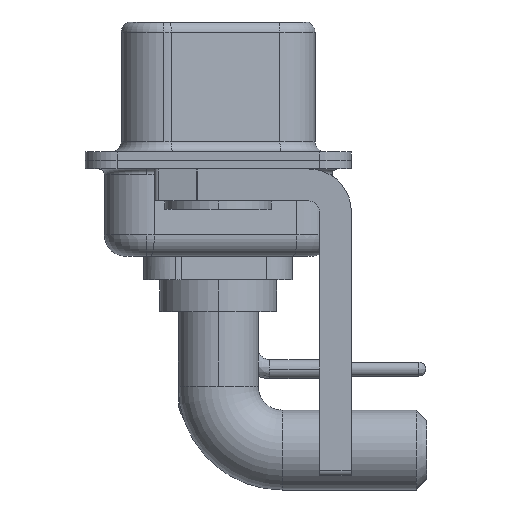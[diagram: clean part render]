
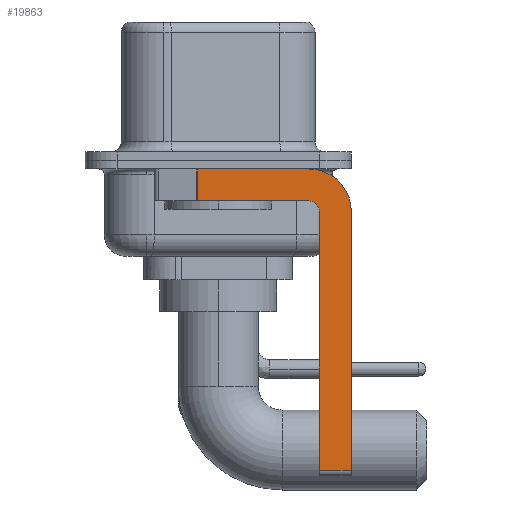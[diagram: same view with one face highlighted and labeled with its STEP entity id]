
A CAD part, left-side view. The second image highlights one B-rep face of the part: STEP entity #19863.
In plain terms, the highlighted planar face has unit normal (-1, 0, 0).
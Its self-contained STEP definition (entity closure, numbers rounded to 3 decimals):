
#294 = DIRECTION ( 'NONE',  ( 1., 0., 0. ) ) ;
#366 = CARTESIAN_POINT ( 'NONE',  ( -2.9, -6.25, -2.4 ) ) ;
#689 = DIRECTION ( 'NONE',  ( 0., 0., -1. ) ) ;
#1173 = VERTEX_POINT ( 'NONE', #2203 ) ;
#1324 = LINE ( 'NONE', #7914, #11558 ) ;
#1544 = VECTOR ( 'NONE', #7559, 1000. ) ;
#1708 = ORIENTED_EDGE ( 'NONE', *, *, #6287, .F. ) ;
#1928 = CARTESIAN_POINT ( 'NONE',  ( -2.9, -4.25, -2.4 ) ) ;
#2134 = CARTESIAN_POINT ( 'NONE',  ( -2.9, 0.978, -0.4 ) ) ;
#2203 = CARTESIAN_POINT ( 'NONE',  ( -2.9, -6.25, -14.55 ) ) ;
#2284 = LINE ( 'NONE', #5813, #1544 ) ;
#2319 = DIRECTION ( 'NONE',  ( 0., -1., 0. ) ) ;
#2606 = EDGE_CURVE ( 'NONE', #8714, #5023, #14496, .T. ) ;
#2607 = EDGE_CURVE ( 'NONE', #15973, #5023, #1324, .T. ) ;
#2671 = DIRECTION ( 'NONE',  ( 1., 0., 0. ) ) ;
#3146 = AXIS2_PLACEMENT_3D ( 'NONE', #1928, #15536, #5555 ) ;
#3405 = EDGE_CURVE ( 'NONE', #16512, #15973, #3497, .T. ) ;
#3497 = CIRCLE ( 'NONE', #3146, 0.5 ) ;
#3884 = CARTESIAN_POINT ( 'NONE',  ( -2.9, 3., -0.4 ) ) ;
#4293 = AXIS2_PLACEMENT_3D ( 'NONE', #10998, #2671, #689 ) ;
#4481 = LINE ( 'NONE', #6443, #9661 ) ;
#5023 = VERTEX_POINT ( 'NONE', #19657 ) ;
#5398 = EDGE_CURVE ( 'NONE', #10180, #1173, #12282, .T. ) ;
#5555 = DIRECTION ( 'NONE',  ( 0., 0., 1. ) ) ;
#5813 = CARTESIAN_POINT ( 'NONE',  ( -2.9, -6.25, -2.4 ) ) ;
#5873 = FACE_OUTER_BOUND ( 'NONE', #6847, .T. ) ;
#6287 = EDGE_CURVE ( 'NONE', #8714, #18024, #12193, .T. ) ;
#6347 = ORIENTED_EDGE ( 'NONE', *, *, #14965, .F. ) ;
#6420 = ORIENTED_EDGE ( 'NONE', *, *, #5398, .T. ) ;
#6443 = CARTESIAN_POINT ( 'NONE',  ( -2.9, -4.75, -14.8 ) ) ;
#6847 = EDGE_LOOP ( 'NONE', ( #1708, #19224, #11988, #19533, #14090, #6420, #12421, #6347 ) ) ;
#6906 = DIRECTION ( 'NONE',  ( 0., 0., -1. ) ) ;
#7509 = CARTESIAN_POINT ( 'NONE',  ( -2.9, -4.75, -14.55 ) ) ;
#7559 = DIRECTION ( 'NONE',  ( 0., 0., -1. ) ) ;
#7914 = CARTESIAN_POINT ( 'NONE',  ( -2.9, -4.25, -1.9 ) ) ;
#8714 = VERTEX_POINT ( 'NONE', #2134 ) ;
#9237 = CARTESIAN_POINT ( 'NONE',  ( -2.9, -4.25, -1.9 ) ) ;
#9661 = VECTOR ( 'NONE', #21037, 1000. ) ;
#9755 = DIRECTION ( 'NONE',  ( 0., 1., 0. ) ) ;
#10180 = VERTEX_POINT ( 'NONE', #7509 ) ;
#10998 = CARTESIAN_POINT ( 'NONE',  ( -2.9, -4.25, -2.4 ) ) ;
#11223 = VECTOR ( 'NONE', #16573, 1000. ) ;
#11558 = VECTOR ( 'NONE', #9755, 1000. ) ;
#11703 = VECTOR ( 'NONE', #2319, 1000. ) ;
#11988 = ORIENTED_EDGE ( 'NONE', *, *, #2607, .F. ) ;
#12193 = LINE ( 'NONE', #3884, #11703 ) ;
#12282 = LINE ( 'NONE', #15802, #19027 ) ;
#12421 = ORIENTED_EDGE ( 'NONE', *, *, #20723, .F. ) ;
#12689 = EDGE_CURVE ( 'NONE', #10180, #16512, #4481, .T. ) ;
#13476 = CARTESIAN_POINT ( 'NONE',  ( -2.9, -4.25, -2.4 ) ) ;
#13923 = DIRECTION ( 'NONE',  ( 0., -1., 0. ) ) ;
#14090 = ORIENTED_EDGE ( 'NONE', *, *, #12689, .F. ) ;
#14496 = LINE ( 'NONE', #16359, #11223 ) ;
#14965 = EDGE_CURVE ( 'NONE', #18024, #19821, #21660, .T. ) ;
#15536 = DIRECTION ( 'NONE',  ( -1., 0., 0. ) ) ;
#15802 = CARTESIAN_POINT ( 'NONE',  ( -2.9, -4.25, -14.55 ) ) ;
#15973 = VERTEX_POINT ( 'NONE', #9237 ) ;
#16359 = CARTESIAN_POINT ( 'NONE',  ( -2.9, 0.978, -1.9 ) ) ;
#16512 = VERTEX_POINT ( 'NONE', #20243 ) ;
#16573 = DIRECTION ( 'NONE',  ( 0., 0., -1. ) ) ;
#17099 = CARTESIAN_POINT ( 'NONE',  ( -2.9, -4.25, -0.4 ) ) ;
#18024 = VERTEX_POINT ( 'NONE', #17099 ) ;
#19027 = VECTOR ( 'NONE', #13923, 1000. ) ;
#19224 = ORIENTED_EDGE ( 'NONE', *, *, #2606, .T. ) ;
#19240 = PLANE ( 'NONE',  #4293 ) ;
#19533 = ORIENTED_EDGE ( 'NONE', *, *, #3405, .F. ) ;
#19573 = AXIS2_PLACEMENT_3D ( 'NONE', #13476, #294, #6906 ) ;
#19657 = CARTESIAN_POINT ( 'NONE',  ( -2.9, 0.978, -1.9 ) ) ;
#19821 = VERTEX_POINT ( 'NONE', #366 ) ;
#19863 = ADVANCED_FACE ( 'NONE', ( #5873 ), #19240, .F. ) ;
#20243 = CARTESIAN_POINT ( 'NONE',  ( -2.9, -4.75, -2.4 ) ) ;
#20723 = EDGE_CURVE ( 'NONE', #19821, #1173, #2284, .T. ) ;
#21037 = DIRECTION ( 'NONE',  ( 0., 0., 1. ) ) ;
#21660 = CIRCLE ( 'NONE', #19573, 2. ) ;
